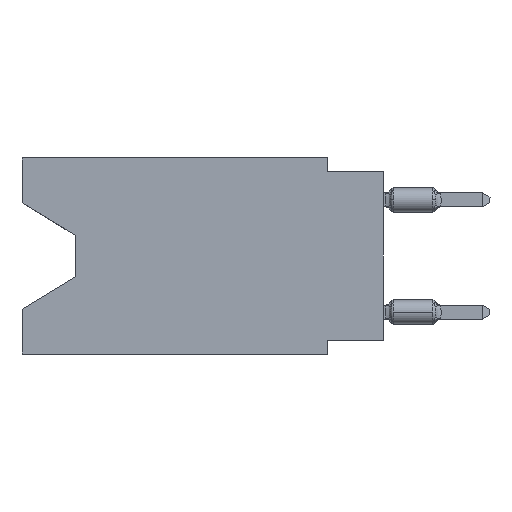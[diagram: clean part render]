
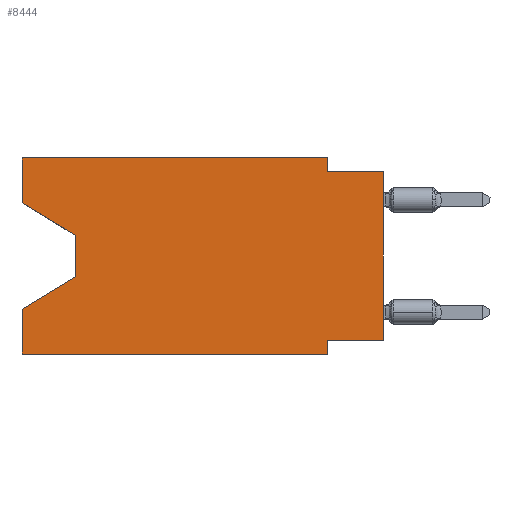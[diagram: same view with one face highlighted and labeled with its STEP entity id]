
A CAD part, left-side view. The second image highlights one B-rep face of the part: STEP entity #8444.
In plain terms, the highlighted planar face has unit normal (-1, 0, 0).
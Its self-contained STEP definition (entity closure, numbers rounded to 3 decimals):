
#166 = EDGE_CURVE ( 'NONE', #19304, #4228, #8161, .T. ) ;
#371 = CARTESIAN_POINT ( 'NONE',  ( 0., 0., -0.635 ) ) ;
#584 = LINE ( 'NONE', #5158, #8630 ) ;
#812 = VECTOR ( 'NONE', #3339, 1000. ) ;
#1030 = CARTESIAN_POINT ( 'NONE',  ( 0., 0., -8.255 ) ) ;
#1037 = ORIENTED_EDGE ( 'NONE', *, *, #13238, .F. ) ;
#1426 = VERTEX_POINT ( 'NONE', #14548 ) ;
#1556 = VERTEX_POINT ( 'NONE', #19518 ) ;
#1592 = CARTESIAN_POINT ( 'NONE',  ( 0., 16.383, 0. ) ) ;
#1604 = EDGE_CURVE ( 'NONE', #1556, #19135, #10658, .T. ) ;
#2062 = EDGE_CURVE ( 'NONE', #15840, #15815, #3245, .T. ) ;
#2122 = VECTOR ( 'NONE', #11495, 1000. ) ;
#2149 = CARTESIAN_POINT ( 'NONE',  ( 0., 16.383, -2.038 ) ) ;
#2258 = ORIENTED_EDGE ( 'NONE', *, *, #12227, .T. ) ;
#2907 = DIRECTION ( 'NONE',  ( 0., 0., -1. ) ) ;
#3078 = ORIENTED_EDGE ( 'NONE', *, *, #19091, .F. ) ;
#3131 = EDGE_LOOP ( 'NONE', ( #12826, #15430, #8290, #1037, #15319, #7415, #4433, #2258, #7048, #7396, #3078, #7198 ) ) ;
#3228 = VERTEX_POINT ( 'NONE', #9915 ) ;
#3245 = LINE ( 'NONE', #16991, #812 ) ;
#3339 = DIRECTION ( 'NONE',  ( 0., 0., 1. ) ) ;
#3972 = EDGE_CURVE ( 'NONE', #7191, #4228, #584, .T. ) ;
#4020 = LINE ( 'NONE', #19373, #11116 ) ;
#4030 = VECTOR ( 'NONE', #13559, 1000. ) ;
#4228 = VERTEX_POINT ( 'NONE', #11650 ) ;
#4433 = ORIENTED_EDGE ( 'NONE', *, *, #19108, .F. ) ;
#4997 = LINE ( 'NONE', #5298, #2122 ) ;
#5096 = CARTESIAN_POINT ( 'NONE',  ( 0., 0., -8.255 ) ) ;
#5158 = CARTESIAN_POINT ( 'NONE',  ( 0., 16.383, -8.89 ) ) ;
#5298 = CARTESIAN_POINT ( 'NONE',  ( 0., 16.383, 0. ) ) ;
#5307 = DIRECTION ( 'NONE',  ( 0., 0.855, -0.519 ) ) ;
#5568 = DIRECTION ( 'NONE',  ( 0., 0., -1. ) ) ;
#5686 = VECTOR ( 'NONE', #2907, 1000. ) ;
#5791 = LINE ( 'NONE', #11870, #5686 ) ;
#5983 = LINE ( 'NONE', #1592, #4030 ) ;
#6129 = VERTEX_POINT ( 'NONE', #15169 ) ;
#7048 = ORIENTED_EDGE ( 'NONE', *, *, #1604, .F. ) ;
#7163 = CARTESIAN_POINT ( 'NONE',  ( 0., 16.383, -8.89 ) ) ;
#7191 = VERTEX_POINT ( 'NONE', #7163 ) ;
#7198 = ORIENTED_EDGE ( 'NONE', *, *, #2062, .F. ) ;
#7202 = DIRECTION ( 'NONE',  ( 0., -0.855, -0.519 ) ) ;
#7396 = ORIENTED_EDGE ( 'NONE', *, *, #13343, .F. ) ;
#7415 = ORIENTED_EDGE ( 'NONE', *, *, #166, .F. ) ;
#7982 = EDGE_CURVE ( 'NONE', #1426, #6129, #4020, .T. ) ;
#8161 = LINE ( 'NONE', #17330, #16828 ) ;
#8264 = DIRECTION ( 'NONE',  ( 0., 0., -1. ) ) ;
#8290 = ORIENTED_EDGE ( 'NONE', *, *, #7982, .T. ) ;
#8444 = ADVANCED_FACE ( 'NONE', ( #13144 ), #19222, .F. ) ;
#8499 = AXIS2_PLACEMENT_3D ( 'NONE', #8569, #14643, #5568 ) ;
#8569 = CARTESIAN_POINT ( 'NONE',  ( 0., 16.383, 0. ) ) ;
#8630 = VECTOR ( 'NONE', #14236, 1000. ) ;
#8710 = LINE ( 'NONE', #14784, #18994 ) ;
#8841 = VECTOR ( 'NONE', #18988, 1000. ) ;
#9717 = CARTESIAN_POINT ( 'NONE',  ( 0., 16.383, 0. ) ) ;
#9915 = CARTESIAN_POINT ( 'NONE',  ( 0., 13.97, -3.505 ) ) ;
#10658 = LINE ( 'NONE', #371, #17872 ) ;
#11116 = VECTOR ( 'NONE', #5307, 1000. ) ;
#11118 = LINE ( 'NONE', #15509, #8841 ) ;
#11144 = LINE ( 'NONE', #18816, #12337 ) ;
#11171 = VERTEX_POINT ( 'NONE', #15097 ) ;
#11433 = VERTEX_POINT ( 'NONE', #1030 ) ;
#11495 = DIRECTION ( 'NONE',  ( 0., -1., 0. ) ) ;
#11650 = CARTESIAN_POINT ( 'NONE',  ( 0., 2.54, -8.89 ) ) ;
#11870 = CARTESIAN_POINT ( 'NONE',  ( 0., 2.54, 0. ) ) ;
#12227 = EDGE_CURVE ( 'NONE', #11433, #19135, #11118, .T. ) ;
#12337 = VECTOR ( 'NONE', #14912, 1000. ) ;
#12826 = ORIENTED_EDGE ( 'NONE', *, *, #19294, .T. ) ;
#12947 = VECTOR ( 'NONE', #14374, 1000. ) ;
#13144 = FACE_OUTER_BOUND ( 'NONE', #3131, .T. ) ;
#13238 = EDGE_CURVE ( 'NONE', #7191, #6129, #5983, .T. ) ;
#13343 = EDGE_CURVE ( 'NONE', #11171, #1556, #5791, .T. ) ;
#13559 = DIRECTION ( 'NONE',  ( 0., 0., 1. ) ) ;
#14236 = DIRECTION ( 'NONE',  ( 0., -1., 0. ) ) ;
#14374 = DIRECTION ( 'NONE',  ( 0., 1., 0. ) ) ;
#14476 = LINE ( 'NONE', #5096, #12947 ) ;
#14548 = CARTESIAN_POINT ( 'NONE',  ( 0., 13.97, -5.385 ) ) ;
#14643 = DIRECTION ( 'NONE',  ( 1., 0., 0. ) ) ;
#14784 = CARTESIAN_POINT ( 'NONE',  ( 0., 16.383, -2.038 ) ) ;
#14912 = DIRECTION ( 'NONE',  ( 0., 0., -1. ) ) ;
#15097 = CARTESIAN_POINT ( 'NONE',  ( 0., 2.54, 0. ) ) ;
#15169 = CARTESIAN_POINT ( 'NONE',  ( 0., 16.383, -6.852 ) ) ;
#15319 = ORIENTED_EDGE ( 'NONE', *, *, #3972, .T. ) ;
#15430 = ORIENTED_EDGE ( 'NONE', *, *, #17084, .T. ) ;
#15509 = CARTESIAN_POINT ( 'NONE',  ( 0., 0., 0. ) ) ;
#15815 = VERTEX_POINT ( 'NONE', #9717 ) ;
#15840 = VERTEX_POINT ( 'NONE', #2149 ) ;
#16828 = VECTOR ( 'NONE', #8264, 1000. ) ;
#16991 = CARTESIAN_POINT ( 'NONE',  ( 0., 16.383, 0. ) ) ;
#17013 = DIRECTION ( 'NONE',  ( 0., -1., 0. ) ) ;
#17084 = EDGE_CURVE ( 'NONE', #3228, #1426, #11144, .T. ) ;
#17330 = CARTESIAN_POINT ( 'NONE',  ( 0., 2.54, -8.89 ) ) ;
#17872 = VECTOR ( 'NONE', #17013, 1000. ) ;
#18346 = CARTESIAN_POINT ( 'NONE',  ( 0., 2.54, -8.255 ) ) ;
#18760 = CARTESIAN_POINT ( 'NONE',  ( 0., 0., -0.635 ) ) ;
#18816 = CARTESIAN_POINT ( 'NONE',  ( 0., 13.97, -3.505 ) ) ;
#18988 = DIRECTION ( 'NONE',  ( 0., 0., 1. ) ) ;
#18994 = VECTOR ( 'NONE', #7202, 1000. ) ;
#19091 = EDGE_CURVE ( 'NONE', #15815, #11171, #4997, .T. ) ;
#19108 = EDGE_CURVE ( 'NONE', #11433, #19304, #14476, .T. ) ;
#19135 = VERTEX_POINT ( 'NONE', #18760 ) ;
#19222 = PLANE ( 'NONE',  #8499 ) ;
#19294 = EDGE_CURVE ( 'NONE', #15840, #3228, #8710, .T. ) ;
#19304 = VERTEX_POINT ( 'NONE', #18346 ) ;
#19373 = CARTESIAN_POINT ( 'NONE',  ( 0., 13.97, -5.385 ) ) ;
#19518 = CARTESIAN_POINT ( 'NONE',  ( 0., 2.54, -0.635 ) ) ;
